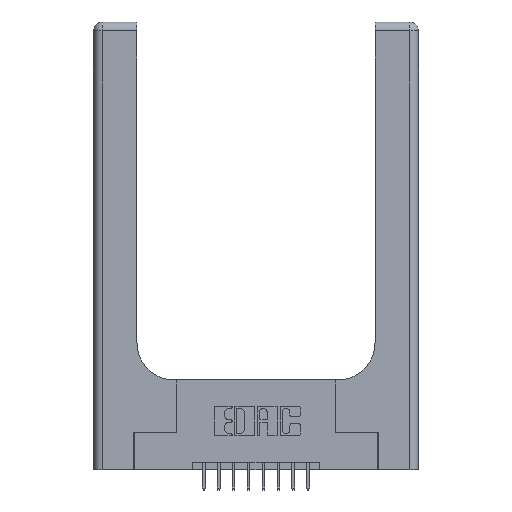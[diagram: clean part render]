
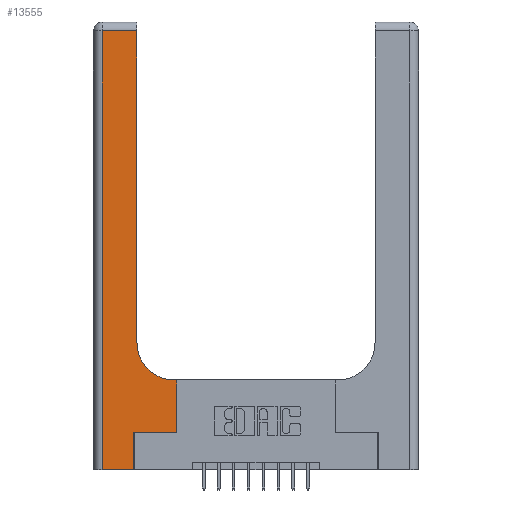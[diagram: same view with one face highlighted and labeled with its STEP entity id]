
A CAD part, top view. The second image highlights one B-rep face of the part: STEP entity #13555.
In plain terms, the highlighted planar face has unit normal (0, 0, 1).
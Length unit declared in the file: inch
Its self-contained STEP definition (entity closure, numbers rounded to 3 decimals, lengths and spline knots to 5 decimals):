
#211 = VERTEX_POINT ( 'NONE', #4445 ) ;
#275 = ORIENTED_EDGE ( 'NONE', *, *, #1581, .T. ) ;
#292 = CARTESIAN_POINT ( 'NONE',  ( 0.269, 0., 0.37 ) ) ;
#530 = VERTEX_POINT ( 'NONE', #2563 ) ;
#583 = EDGE_CURVE ( 'NONE', #2498, #976, #1495, .T. ) ;
#637 = CIRCLE ( 'NONE', #900, 0.25 ) ;
#779 = CARTESIAN_POINT ( 'NONE',  ( 0., 3., 0.37 ) ) ;
#900 = AXIS2_PLACEMENT_3D ( 'NONE', #5777, #5859, #3390 ) ;
#976 = VERTEX_POINT ( 'NONE', #13717 ) ;
#1495 = LINE ( 'NONE', #292, #4314 ) ;
#1581 = EDGE_CURVE ( 'NONE', #211, #8785, #12853, .T. ) ;
#1657 = CARTESIAN_POINT ( 'NONE',  ( 0.2915, 0.6, 0.37 ) ) ;
#2116 = DIRECTION ( 'NONE',  ( 0., -1., 0. ) ) ;
#2257 = VECTOR ( 'NONE', #9264, 39.37008 ) ;
#2422 = ORIENTED_EDGE ( 'NONE', *, *, #3610, .T. ) ;
#2498 = VERTEX_POINT ( 'NONE', #5843 ) ;
#2505 = VECTOR ( 'NONE', #13866, 39.37008 ) ;
#2563 = CARTESIAN_POINT ( 'NONE',  ( 0.5585, 0.25, 0.37 ) ) ;
#2651 = LINE ( 'NONE', #9131, #2505 ) ;
#3390 = DIRECTION ( 'NONE',  ( 1., 0., 0. ) ) ;
#3404 = VECTOR ( 'NONE', #2116, 39.37008 ) ;
#3610 = EDGE_CURVE ( 'NONE', #3611, #2498, #8397, .T. ) ;
#3611 = VERTEX_POINT ( 'NONE', #10621 ) ;
#3864 = EDGE_CURVE ( 'NONE', #976, #530, #2651, .T. ) ;
#4314 = VECTOR ( 'NONE', #5247, 39.37008 ) ;
#4445 = CARTESIAN_POINT ( 'NONE',  ( 0.2915, 0.85, 0.37 ) ) ;
#4580 = LINE ( 'NONE', #12199, #8717 ) ;
#4931 = EDGE_LOOP ( 'NONE', ( #275, #12097, #8346, #2422, #10431, #13919, #14027, #5772, #14569 ) ) ;
#4969 = VERTEX_POINT ( 'NONE', #10287 ) ;
#5093 = CARTESIAN_POINT ( 'NONE',  ( 0.5585, 0.6, 0.37 ) ) ;
#5247 = DIRECTION ( 'NONE',  ( 0., 1., 0. ) ) ;
#5496 = CARTESIAN_POINT ( 'NONE',  ( 0., 2.94, 0.37 ) ) ;
#5720 = LINE ( 'NONE', #15699, #3404 ) ;
#5727 = DIRECTION ( 'NONE',  ( 0., 1., 0. ) ) ;
#5754 = DIRECTION ( 'NONE',  ( -1., 0., 0. ) ) ;
#5772 = ORIENTED_EDGE ( 'NONE', *, *, #9343, .T. ) ;
#5777 = CARTESIAN_POINT ( 'NONE',  ( 0.5415, 0.85, 0.37 ) ) ;
#5843 = CARTESIAN_POINT ( 'NONE',  ( 0.269, 0., 0.37 ) ) ;
#5847 = DIRECTION ( 'NONE',  ( 1., 0., 0. ) ) ;
#5859 = DIRECTION ( 'NONE',  ( 0., 0., -1. ) ) ;
#6038 = VERTEX_POINT ( 'NONE', #15735 ) ;
#6818 = LINE ( 'NONE', #1657, #14948 ) ;
#7249 = PLANE ( 'NONE',  #13710 ) ;
#7997 = EDGE_CURVE ( 'NONE', #4969, #3611, #5720, .T. ) ;
#8154 = CARTESIAN_POINT ( 'NONE',  ( 0., 0., 0.37 ) ) ;
#8346 = ORIENTED_EDGE ( 'NONE', *, *, #7997, .T. ) ;
#8397 = LINE ( 'NONE', #8154, #15083 ) ;
#8717 = VECTOR ( 'NONE', #5727, 39.37008 ) ;
#8785 = VERTEX_POINT ( 'NONE', #14485 ) ;
#9131 = CARTESIAN_POINT ( 'NONE',  ( 0.269, 0.25, 0.37 ) ) ;
#9199 = LINE ( 'NONE', #5496, #10874 ) ;
#9264 = DIRECTION ( 'NONE',  ( 0., 1., 0. ) ) ;
#9343 = EDGE_CURVE ( 'NONE', #14796, #6038, #6818, .T. ) ;
#9978 = EDGE_CURVE ( 'NONE', #530, #14796, #4580, .T. ) ;
#10287 = CARTESIAN_POINT ( 'NONE',  ( 0.06, 2.94, 0.37 ) ) ;
#10356 = DIRECTION ( 'NONE',  ( -1., 0., 0. ) ) ;
#10431 = ORIENTED_EDGE ( 'NONE', *, *, #583, .T. ) ;
#10600 = DIRECTION ( 'NONE',  ( -1., 0., 0. ) ) ;
#10621 = CARTESIAN_POINT ( 'NONE',  ( 0.06, 0., 0.37 ) ) ;
#10874 = VECTOR ( 'NONE', #10356, 39.37008 ) ;
#11984 = FACE_OUTER_BOUND ( 'NONE', #4931, .T. ) ;
#12097 = ORIENTED_EDGE ( 'NONE', *, *, #14988, .T. ) ;
#12199 = CARTESIAN_POINT ( 'NONE',  ( 0.5585, 0.25, 0.37 ) ) ;
#12853 = LINE ( 'NONE', #15387, #2257 ) ;
#13253 = EDGE_CURVE ( 'NONE', #6038, #211, #637, .T. ) ;
#13555 = ADVANCED_FACE ( 'NONE', ( #11984 ), #7249, .F. ) ;
#13710 = AXIS2_PLACEMENT_3D ( 'NONE', #779, #14663, #5754 ) ;
#13717 = CARTESIAN_POINT ( 'NONE',  ( 0.269, 0.25, 0.37 ) ) ;
#13866 = DIRECTION ( 'NONE',  ( 1., 0., 0. ) ) ;
#13919 = ORIENTED_EDGE ( 'NONE', *, *, #3864, .T. ) ;
#14027 = ORIENTED_EDGE ( 'NONE', *, *, #9978, .T. ) ;
#14485 = CARTESIAN_POINT ( 'NONE',  ( 0.2915, 2.94, 0.37 ) ) ;
#14569 = ORIENTED_EDGE ( 'NONE', *, *, #13253, .T. ) ;
#14663 = DIRECTION ( 'NONE',  ( 0., 0., -1. ) ) ;
#14796 = VERTEX_POINT ( 'NONE', #5093 ) ;
#14948 = VECTOR ( 'NONE', #10600, 39.37008 ) ;
#14988 = EDGE_CURVE ( 'NONE', #8785, #4969, #9199, .T. ) ;
#15083 = VECTOR ( 'NONE', #5847, 39.37008 ) ;
#15387 = CARTESIAN_POINT ( 'NONE',  ( 0.2915, 3., 0.37 ) ) ;
#15699 = CARTESIAN_POINT ( 'NONE',  ( 0.06, 3., 0.37 ) ) ;
#15735 = CARTESIAN_POINT ( 'NONE',  ( 0.5415, 0.6, 0.37 ) ) ;
